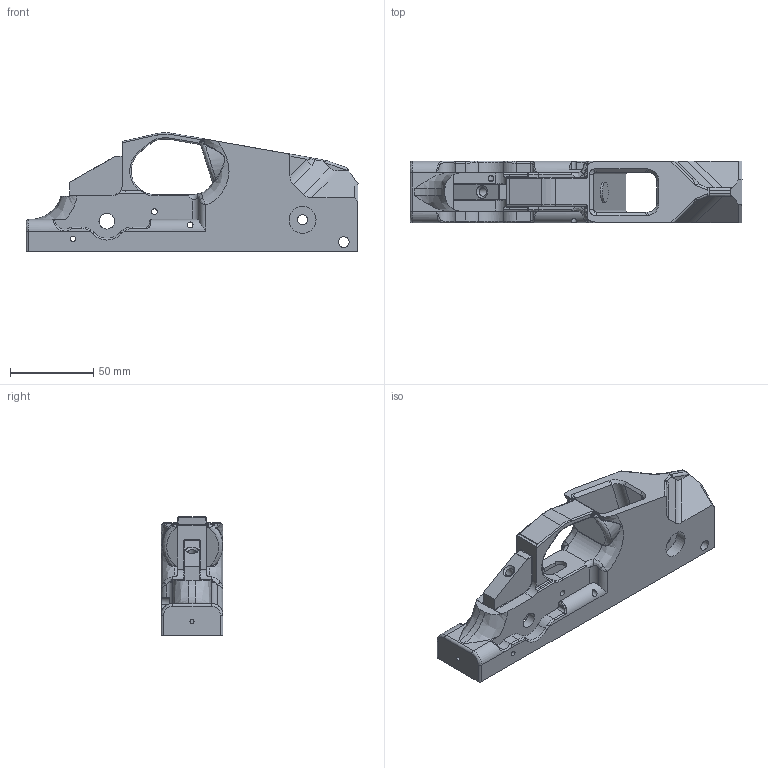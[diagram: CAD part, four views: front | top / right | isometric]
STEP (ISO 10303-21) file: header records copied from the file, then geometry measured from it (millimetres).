
FILE_DESCRIPTION (( 'STEP AP203' ), '1' );
FILE_NAME ('WTF-9MV_lower_receiver-BLANK.STEP', '2020-05-14T02:59:49', ( '' ), ( '' ), 'SwSTEP 2.0', 'SolidWorks 2016', '' );
FILE_SCHEMA (( 'CONFIG_CONTROL_DESIGN' ));
Length unit declared in the file: millimetre
Products named in the file (1): WTF-9MV_lower_receiver-BLANK
Bounding box: 199.47 x 37.13 x 71.26 mm (x, y, z)
Volume: 192614.2 mm3; surface area: 54429.2 mm2
Topology: 2 solids, 2 shells, 366 faces, 988 edges, 613 vertices
Faces by surface type: cylinder 142, bspline 116, plane 105, cone 2, torus 1
Full cylindrical faces by diameter (mm): 2.5 x1, 3 x1, 3.175 x3, 3.469 x4, 5.105 x1, 6 x1, 6.4 x2, 8 x1, 9.525 x2, 12 x1, 16.2 x1
Entity records: 19204 total; most frequent: CARTESIAN_POINT 11229, ORIENTED_EDGE 1892, DIRECTION 1233, EDGE_CURVE 946, VERTEX_POINT 603, AXIS2_PLACEMENT_3D 425, EDGE_LOOP 419, FACE_OUTER_BOUND 385
